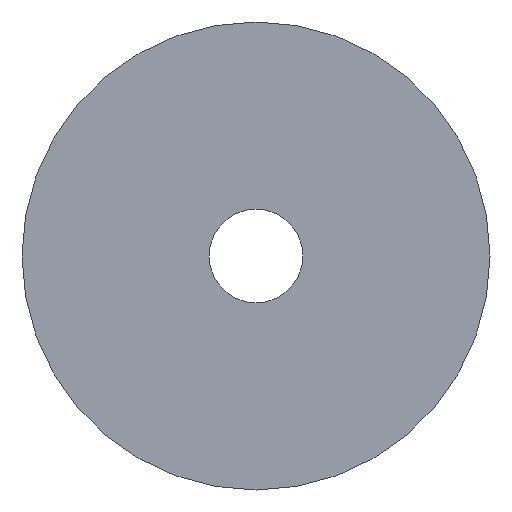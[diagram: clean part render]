
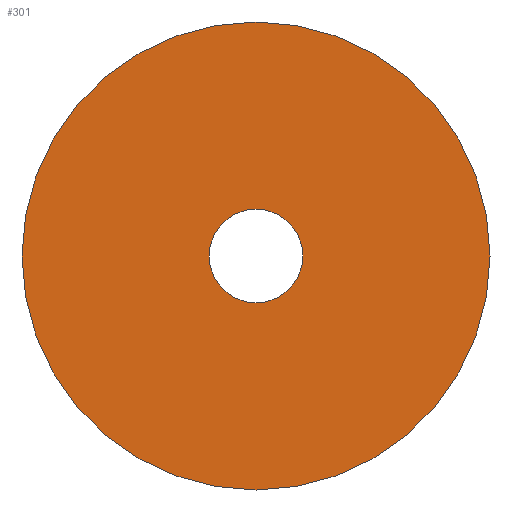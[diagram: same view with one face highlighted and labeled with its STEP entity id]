
A CAD part, front view. The second image highlights one B-rep face of the part: STEP entity #301.
In plain terms, the highlighted planar face has unit normal (0, -1, 0).
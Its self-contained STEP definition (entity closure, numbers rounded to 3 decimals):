
#15 = VERTEX_POINT ( 'NONE', #159 ) ;
#17 = VERTEX_POINT ( 'NONE', #158 ) ;
#26 = EDGE_LOOP ( 'NONE', ( #209, #205 ) ) ;
#36 = ORIENTED_EDGE ( 'NONE', *, *, #272, .T. ) ;
#56 = DIRECTION ( 'NONE',  ( 0., 0., -1. ) ) ;
#57 = DIRECTION ( 'NONE',  ( 0., -1., 0. ) ) ;
#61 = CARTESIAN_POINT ( 'NONE',  ( 0., 0., 0. ) ) ;
#102 = DIRECTION ( 'NONE',  ( 0., 0., -1. ) ) ;
#103 = DIRECTION ( 'NONE',  ( 0., -1., 0. ) ) ;
#104 = CARTESIAN_POINT ( 'NONE',  ( 1.5, 0., 0. ) ) ;
#105 = PLANE ( 'NONE',  #255 ) ;
#127 = DIRECTION ( 'NONE',  ( 0., 0., -1. ) ) ;
#128 = DIRECTION ( 'NONE',  ( 0., -1., 0. ) ) ;
#129 = CARTESIAN_POINT ( 'NONE',  ( 0., 0., 0. ) ) ;
#133 = DIRECTION ( 'NONE',  ( 0., 0., -1. ) ) ;
#134 = DIRECTION ( 'NONE',  ( 0., -1., 0. ) ) ;
#138 = CARTESIAN_POINT ( 'NONE',  ( 0., 0., 0. ) ) ;
#142 = DIRECTION ( 'NONE',  ( 0., 0., -1. ) ) ;
#143 = DIRECTION ( 'NONE',  ( 0., -1., 0. ) ) ;
#144 = CARTESIAN_POINT ( 'NONE',  ( 0., 0., 0. ) ) ;
#150 = CARTESIAN_POINT ( 'NONE',  ( 0., 0., -7.5 ) ) ;
#151 = CARTESIAN_POINT ( 'NONE',  ( 0., 0., 7.5 ) ) ;
#158 = CARTESIAN_POINT ( 'NONE',  ( 0., 0., -1.5 ) ) ;
#159 = CARTESIAN_POINT ( 'NONE',  ( 0., 0., 1.5 ) ) ;
#175 = VERTEX_POINT ( 'NONE', #151 ) ;
#176 = VERTEX_POINT ( 'NONE', #150 ) ;
#198 = ORIENTED_EDGE ( 'NONE', *, *, #316, .T. ) ;
#200 = EDGE_LOOP ( 'NONE', ( #198, #36 ) ) ;
#205 = ORIENTED_EDGE ( 'NONE', *, *, #274, .F. ) ;
#209 = ORIENTED_EDGE ( 'NONE', *, *, #268, .F. ) ;
#211 = AXIS2_PLACEMENT_3D ( 'NONE', #138, #134, #133 ) ;
#215 = AXIS2_PLACEMENT_3D ( 'NONE', #129, #128, #127 ) ;
#238 = AXIS2_PLACEMENT_3D ( 'NONE', #61, #57, #56 ) ;
#255 = AXIS2_PLACEMENT_3D ( 'NONE', #104, #103, #102 ) ;
#258 = FACE_BOUND ( 'NONE', #26, .T. ) ;
#263 = FACE_OUTER_BOUND ( 'NONE', #200, .T. ) ;
#265 = AXIS2_PLACEMENT_3D ( 'NONE', #144, #143, #142 ) ;
#268 = EDGE_CURVE ( 'NONE', #17, #15, #294, .T. ) ;
#269 = CIRCLE ( 'NONE', #211, 7.5 ) ;
#272 = EDGE_CURVE ( 'NONE', #175, #176, #269, .T. ) ;
#274 = EDGE_CURVE ( 'NONE', #15, #17, #295, .T. ) ;
#281 = CIRCLE ( 'NONE', #238, 7.5 ) ;
#294 = CIRCLE ( 'NONE', #265, 1.5 ) ;
#295 = CIRCLE ( 'NONE', #215, 1.5 ) ;
#301 = ADVANCED_FACE ( 'NONE', ( #263, #258 ), #105, .T. ) ;
#316 = EDGE_CURVE ( 'NONE', #176, #175, #281, .T. ) ;
